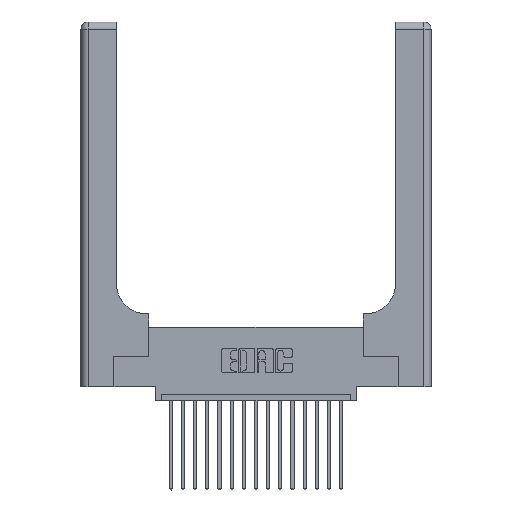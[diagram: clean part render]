
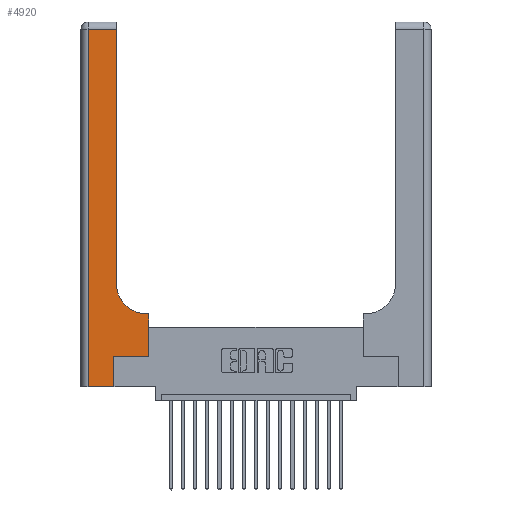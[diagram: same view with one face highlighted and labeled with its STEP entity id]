
A CAD part, top view. The second image highlights one B-rep face of the part: STEP entity #4920.
In plain terms, the highlighted planar face has unit normal (0, 0, 1).
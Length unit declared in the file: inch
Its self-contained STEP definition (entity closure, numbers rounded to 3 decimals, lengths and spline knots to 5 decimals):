
#17 = LINE ( 'NONE', #5363, #16206 ) ;
#211 = CARTESIAN_POINT ( 'NONE',  ( 0.06, 3., 0.37 ) ) ;
#734 = ORIENTED_EDGE ( 'NONE', *, *, #3276, .T. ) ;
#1114 = VERTEX_POINT ( 'NONE', #9580 ) ;
#1181 = DIRECTION ( 'NONE',  ( -1., 0., 0. ) ) ;
#1379 = PLANE ( 'NONE',  #7408 ) ;
#1408 = LINE ( 'NONE', #8076, #19762 ) ;
#1672 = VERTEX_POINT ( 'NONE', #12658 ) ;
#2140 = CARTESIAN_POINT ( 'NONE',  ( 0.5585, 0.6, 0.37 ) ) ;
#2401 = VECTOR ( 'NONE', #6813, 39.37008 ) ;
#2686 = DIRECTION ( 'NONE',  ( -1., 0., 0. ) ) ;
#2724 = VERTEX_POINT ( 'NONE', #15604 ) ;
#2946 = CARTESIAN_POINT ( 'NONE',  ( 0.2915, 0.6, 0.37 ) ) ;
#3276 = EDGE_CURVE ( 'NONE', #6508, #11386, #1408, .T. ) ;
#3776 = CARTESIAN_POINT ( 'NONE',  ( 0.2915, 2.94, 0.37 ) ) ;
#4184 = VERTEX_POINT ( 'NONE', #3776 ) ;
#4920 = ADVANCED_FACE ( 'NONE', ( #8052 ), #1379, .F. ) ;
#5363 = CARTESIAN_POINT ( 'NONE',  ( 0.269, 0., 0.37 ) ) ;
#5391 = LINE ( 'NONE', #12906, #13237 ) ;
#5739 = CARTESIAN_POINT ( 'NONE',  ( 0.5585, 0.25, 0.37 ) ) ;
#6365 = ORIENTED_EDGE ( 'NONE', *, *, #16428, .T. ) ;
#6508 = VERTEX_POINT ( 'NONE', #5739 ) ;
#6813 = DIRECTION ( 'NONE',  ( 1., 0., 0. ) ) ;
#7179 = EDGE_CURVE ( 'NONE', #9588, #13153, #18488, .T. ) ;
#7408 = AXIS2_PLACEMENT_3D ( 'NONE', #18181, #15361, #1181 ) ;
#7674 = CIRCLE ( 'NONE', #10862, 0.25 ) ;
#7696 = LINE ( 'NONE', #19865, #12841 ) ;
#7867 = EDGE_CURVE ( 'NONE', #4184, #2724, #7696, .T. ) ;
#8052 = FACE_OUTER_BOUND ( 'NONE', #18836, .T. ) ;
#8076 = CARTESIAN_POINT ( 'NONE',  ( 0.5585, 0.25, 0.37 ) ) ;
#8963 = EDGE_CURVE ( 'NONE', #1672, #1114, #7674, .T. ) ;
#9263 = LINE ( 'NONE', #13244, #2401 ) ;
#9293 = ORIENTED_EDGE ( 'NONE', *, *, #18658, .T. ) ;
#9580 = CARTESIAN_POINT ( 'NONE',  ( 0.2915, 0.85, 0.37 ) ) ;
#9588 = VERTEX_POINT ( 'NONE', #13488 ) ;
#9608 = ORIENTED_EDGE ( 'NONE', *, *, #8963, .T. ) ;
#10161 = ORIENTED_EDGE ( 'NONE', *, *, #15373, .T. ) ;
#10862 = AXIS2_PLACEMENT_3D ( 'NONE', #16888, #12179, #12043 ) ;
#11152 = VECTOR ( 'NONE', #11269, 39.37008 ) ;
#11163 = DIRECTION ( 'NONE',  ( 0., 1., 0. ) ) ;
#11172 = DIRECTION ( 'NONE',  ( 0., -1., 0. ) ) ;
#11173 = DIRECTION ( 'NONE',  ( 0., 1., 0. ) ) ;
#11269 = DIRECTION ( 'NONE',  ( 1., 0., 0. ) ) ;
#11386 = VERTEX_POINT ( 'NONE', #2140 ) ;
#11997 = VECTOR ( 'NONE', #18622, 39.37008 ) ;
#12043 = DIRECTION ( 'NONE',  ( 1., 0., 0. ) ) ;
#12179 = DIRECTION ( 'NONE',  ( 0., 0., -1. ) ) ;
#12658 = CARTESIAN_POINT ( 'NONE',  ( 0.5415, 0.6, 0.37 ) ) ;
#12736 = ORIENTED_EDGE ( 'NONE', *, *, #18235, .T. ) ;
#12841 = VECTOR ( 'NONE', #2686, 39.37008 ) ;
#12906 = CARTESIAN_POINT ( 'NONE',  ( 0.2915, 3., 0.37 ) ) ;
#13153 = VERTEX_POINT ( 'NONE', #17454 ) ;
#13237 = VECTOR ( 'NONE', #11163, 39.37008 ) ;
#13244 = CARTESIAN_POINT ( 'NONE',  ( 0.269, 0.25, 0.37 ) ) ;
#13488 = CARTESIAN_POINT ( 'NONE',  ( 0.06, 0., 0.37 ) ) ;
#13661 = ORIENTED_EDGE ( 'NONE', *, *, #14686, .T. ) ;
#14356 = CARTESIAN_POINT ( 'NONE',  ( 0., 0., 0.37 ) ) ;
#14686 = EDGE_CURVE ( 'NONE', #1114, #4184, #5391, .T. ) ;
#15361 = DIRECTION ( 'NONE',  ( 0., 0., -1. ) ) ;
#15373 = EDGE_CURVE ( 'NONE', #19186, #6508, #9263, .T. ) ;
#15604 = CARTESIAN_POINT ( 'NONE',  ( 0.06, 2.94, 0.37 ) ) ;
#15814 = CARTESIAN_POINT ( 'NONE',  ( 0.269, 0.25, 0.37 ) ) ;
#16206 = VECTOR ( 'NONE', #19261, 39.37008 ) ;
#16347 = VECTOR ( 'NONE', #11172, 39.37008 ) ;
#16428 = EDGE_CURVE ( 'NONE', #2724, #9588, #19977, .T. ) ;
#16888 = CARTESIAN_POINT ( 'NONE',  ( 0.5415, 0.85, 0.37 ) ) ;
#17454 = CARTESIAN_POINT ( 'NONE',  ( 0.269, 0., 0.37 ) ) ;
#17543 = ORIENTED_EDGE ( 'NONE', *, *, #7179, .T. ) ;
#17640 = ORIENTED_EDGE ( 'NONE', *, *, #7867, .T. ) ;
#18181 = CARTESIAN_POINT ( 'NONE',  ( 0., 3., 0.37 ) ) ;
#18235 = EDGE_CURVE ( 'NONE', #13153, #19186, #17, .T. ) ;
#18488 = LINE ( 'NONE', #14356, #11152 ) ;
#18622 = DIRECTION ( 'NONE',  ( -1., 0., 0. ) ) ;
#18658 = EDGE_CURVE ( 'NONE', #11386, #1672, #18833, .T. ) ;
#18833 = LINE ( 'NONE', #2946, #11997 ) ;
#18836 = EDGE_LOOP ( 'NONE', ( #13661, #17640, #6365, #17543, #12736, #10161, #734, #9293, #9608 ) ) ;
#19186 = VERTEX_POINT ( 'NONE', #15814 ) ;
#19261 = DIRECTION ( 'NONE',  ( 0., 1., 0. ) ) ;
#19762 = VECTOR ( 'NONE', #11173, 39.37008 ) ;
#19865 = CARTESIAN_POINT ( 'NONE',  ( 0., 2.94, 0.37 ) ) ;
#19977 = LINE ( 'NONE', #211, #16347 ) ;
